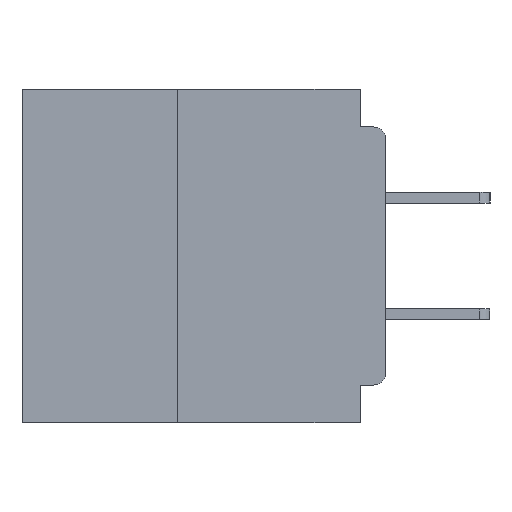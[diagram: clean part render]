
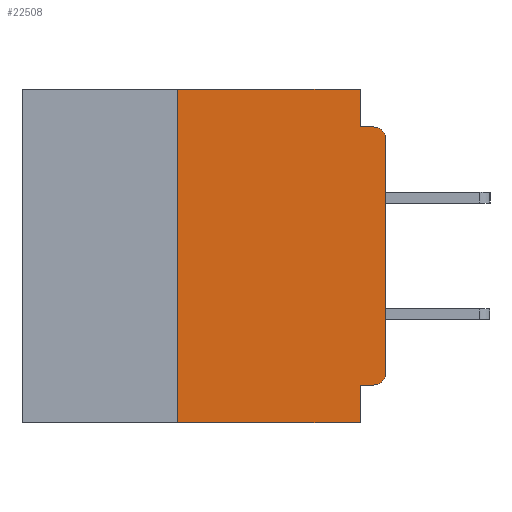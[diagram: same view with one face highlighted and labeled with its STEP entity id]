
A CAD part, left-side view. The second image highlights one B-rep face of the part: STEP entity #22508.
In plain terms, the highlighted planar face has unit normal (-1, 0, 0).
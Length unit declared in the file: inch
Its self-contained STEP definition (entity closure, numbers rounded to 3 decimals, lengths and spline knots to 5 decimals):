
#130 = DIRECTION ( 'NONE',  ( 0., -1., 0. ) ) ;
#429 = EDGE_LOOP ( 'NONE', ( #36731, #13284, #34451, #9081, #8859, #28454, #1526, #8648, #1393, #17977 ) ) ;
#759 = LINE ( 'NONE', #12540, #8854 ) ;
#1393 = ORIENTED_EDGE ( 'NONE', *, *, #31714, .F. ) ;
#1526 = ORIENTED_EDGE ( 'NONE', *, *, #38693, .T. ) ;
#2028 = AXIS2_PLACEMENT_3D ( 'NONE', #20540, #11565, #32641 ) ;
#2289 = CARTESIAN_POINT ( 'NONE',  ( 0., 0.25, 0. ) ) ;
#2882 = LINE ( 'NONE', #24559, #34033 ) ;
#3062 = VERTEX_POINT ( 'NONE', #29295 ) ;
#3101 = DIRECTION ( 'NONE',  ( 0., -1., 0. ) ) ;
#3111 = CARTESIAN_POINT ( 'NONE',  ( 0., 0.015, -0.06 ) ) ;
#3190 = CARTESIAN_POINT ( 'NONE',  ( 0., 0.25, -0.4 ) ) ;
#3627 = VERTEX_POINT ( 'NONE', #37758 ) ;
#5145 = LINE ( 'NONE', #18236, #13259 ) ;
#5306 = VECTOR ( 'NONE', #130, 39.37008 ) ;
#5915 = DIRECTION ( 'NONE',  ( 0., 0., 1. ) ) ;
#6181 = DIRECTION ( 'NONE',  ( 0., 0., -1. ) ) ;
#6492 = CARTESIAN_POINT ( 'NONE',  ( 0., 0., -0.045 ) ) ;
#7149 = AXIS2_PLACEMENT_3D ( 'NONE', #25734, #7563, #28741 ) ;
#7563 = DIRECTION ( 'NONE',  ( -1., 0., 0. ) ) ;
#8648 = ORIENTED_EDGE ( 'NONE', *, *, #13405, .F. ) ;
#8854 = VECTOR ( 'NONE', #15586, 39.37008 ) ;
#8859 = ORIENTED_EDGE ( 'NONE', *, *, #22133, .F. ) ;
#9081 = ORIENTED_EDGE ( 'NONE', *, *, #20068, .F. ) ;
#10081 = FACE_OUTER_BOUND ( 'NONE', #429, .T. ) ;
#10122 = EDGE_CURVE ( 'NONE', #15165, #26217, #34981, .T. ) ;
#10567 = CARTESIAN_POINT ( 'NONE',  ( 0., 0.031, -0.4 ) ) ;
#11194 = VERTEX_POINT ( 'NONE', #11586 ) ;
#11565 = DIRECTION ( 'NONE',  ( 1., 0., 0. ) ) ;
#11586 = CARTESIAN_POINT ( 'NONE',  ( 0., 0.25, -0.4 ) ) ;
#12540 = CARTESIAN_POINT ( 'NONE',  ( 0., 0.031, 0. ) ) ;
#12802 = VERTEX_POINT ( 'NONE', #37876 ) ;
#13074 = EDGE_CURVE ( 'NONE', #12802, #15165, #33333, .T. ) ;
#13109 = VECTOR ( 'NONE', #31662, 39.37008 ) ;
#13259 = VECTOR ( 'NONE', #3101, 39.37008 ) ;
#13284 = ORIENTED_EDGE ( 'NONE', *, *, #10122, .T. ) ;
#13405 = EDGE_CURVE ( 'NONE', #34442, #15614, #28226, .T. ) ;
#14152 = CARTESIAN_POINT ( 'NONE',  ( 0., 0.031, -0.355 ) ) ;
#14283 = CIRCLE ( 'NONE', #7149, 0.015 ) ;
#14363 = LINE ( 'NONE', #6492, #21449 ) ;
#15042 = EDGE_CURVE ( 'NONE', #3062, #26217, #14363, .T. ) ;
#15165 = VERTEX_POINT ( 'NONE', #22134 ) ;
#15273 = CARTESIAN_POINT ( 'NONE',  ( 0., 0.437, 0. ) ) ;
#15586 = DIRECTION ( 'NONE',  ( 0., 0., -1. ) ) ;
#15614 = VERTEX_POINT ( 'NONE', #33208 ) ;
#17977 = ORIENTED_EDGE ( 'NONE', *, *, #23701, .T. ) ;
#18236 = CARTESIAN_POINT ( 'NONE',  ( 0., 0.437, -0.4 ) ) ;
#19622 = CARTESIAN_POINT ( 'NONE',  ( 0., 0.031, 0. ) ) ;
#20068 = EDGE_CURVE ( 'NONE', #31444, #3062, #759, .T. ) ;
#20540 = CARTESIAN_POINT ( 'NONE',  ( 0., 0.437, 0. ) ) ;
#21449 = VECTOR ( 'NONE', #27692, 39.37008 ) ;
#21982 = VERTEX_POINT ( 'NONE', #2289 ) ;
#22133 = EDGE_CURVE ( 'NONE', #21982, #31444, #37304, .T. ) ;
#22134 = CARTESIAN_POINT ( 'NONE',  ( 0., 0., -0.06 ) ) ;
#22154 = EDGE_CURVE ( 'NONE', #11194, #21982, #36379, .T. ) ;
#22508 = ADVANCED_FACE ( 'NONE', ( #10081 ), #29647, .F. ) ;
#23701 = EDGE_CURVE ( 'NONE', #3627, #12802, #14283, .T. ) ;
#24097 = CARTESIAN_POINT ( 'NONE',  ( 0., 0., 0. ) ) ;
#24368 = DIRECTION ( 'NONE',  ( -1., 0., 0. ) ) ;
#24559 = CARTESIAN_POINT ( 'NONE',  ( 0., 0., -0.355 ) ) ;
#25734 = CARTESIAN_POINT ( 'NONE',  ( 0., 0.015, -0.34 ) ) ;
#26217 = VERTEX_POINT ( 'NONE', #37144 ) ;
#26408 = VECTOR ( 'NONE', #5915, 39.37008 ) ;
#27440 = DIRECTION ( 'NONE',  ( 0., 0., 1. ) ) ;
#27692 = DIRECTION ( 'NONE',  ( 0., -1., 0. ) ) ;
#27699 = DIRECTION ( 'NONE',  ( 0., 1., 0. ) ) ;
#28151 = AXIS2_PLACEMENT_3D ( 'NONE', #3111, #24368, #6181 ) ;
#28226 = LINE ( 'NONE', #10567, #13109 ) ;
#28454 = ORIENTED_EDGE ( 'NONE', *, *, #22154, .F. ) ;
#28547 = VECTOR ( 'NONE', #27440, 39.37008 ) ;
#28741 = DIRECTION ( 'NONE',  ( 0., 0., -1. ) ) ;
#29295 = CARTESIAN_POINT ( 'NONE',  ( 0., 0.031, -0.045 ) ) ;
#29647 = PLANE ( 'NONE',  #2028 ) ;
#31444 = VERTEX_POINT ( 'NONE', #19622 ) ;
#31662 = DIRECTION ( 'NONE',  ( 0., 0., -1. ) ) ;
#31714 = EDGE_CURVE ( 'NONE', #3627, #34442, #2882, .T. ) ;
#32641 = DIRECTION ( 'NONE',  ( 0., 0., -1. ) ) ;
#33208 = CARTESIAN_POINT ( 'NONE',  ( 0., 0.031, -0.4 ) ) ;
#33333 = LINE ( 'NONE', #24097, #26408 ) ;
#34033 = VECTOR ( 'NONE', #27699, 39.37008 ) ;
#34442 = VERTEX_POINT ( 'NONE', #14152 ) ;
#34451 = ORIENTED_EDGE ( 'NONE', *, *, #15042, .F. ) ;
#34981 = CIRCLE ( 'NONE', #28151, 0.015 ) ;
#36379 = LINE ( 'NONE', #3190, #28547 ) ;
#36731 = ORIENTED_EDGE ( 'NONE', *, *, #13074, .T. ) ;
#37144 = CARTESIAN_POINT ( 'NONE',  ( 0., 0.015, -0.045 ) ) ;
#37304 = LINE ( 'NONE', #15273, #5306 ) ;
#37758 = CARTESIAN_POINT ( 'NONE',  ( 0., 0.015, -0.355 ) ) ;
#37876 = CARTESIAN_POINT ( 'NONE',  ( 0., 0., -0.34 ) ) ;
#38693 = EDGE_CURVE ( 'NONE', #11194, #15614, #5145, .T. ) ;
